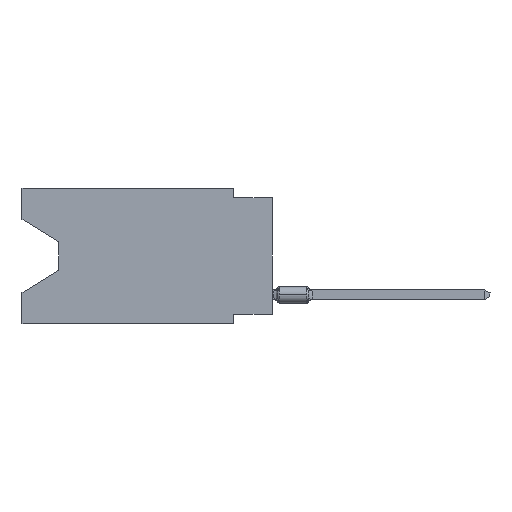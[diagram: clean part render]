
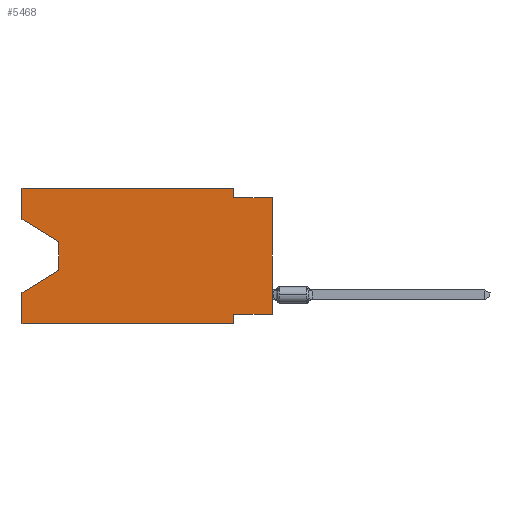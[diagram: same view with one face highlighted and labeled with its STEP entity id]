
A CAD part, left-side view. The second image highlights one B-rep face of the part: STEP entity #5468.
In plain terms, the highlighted planar face has unit normal (-1, 0, 0).
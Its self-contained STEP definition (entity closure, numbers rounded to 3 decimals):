
#30 = DIRECTION ( 'NONE',  ( 0., 0., -1. ) ) ;
#719 = CARTESIAN_POINT ( 'NONE',  ( 0., 0., -0.635 ) ) ;
#781 = CARTESIAN_POINT ( 'NONE',  ( 0., 16.383, -8.89 ) ) ;
#1116 = CARTESIAN_POINT ( 'NONE',  ( 0., 0., -0.635 ) ) ;
#1270 = DIRECTION ( 'NONE',  ( 0., 0., 1. ) ) ;
#1694 = VERTEX_POINT ( 'NONE', #15771 ) ;
#2422 = EDGE_CURVE ( 'NONE', #11921, #3407, #35065, .T. ) ;
#2826 = LINE ( 'NONE', #18841, #31765 ) ;
#3257 = CARTESIAN_POINT ( 'NONE',  ( 0., 13.97, -5.385 ) ) ;
#3407 = VERTEX_POINT ( 'NONE', #30280 ) ;
#3921 = LINE ( 'NONE', #30478, #16487 ) ;
#4102 = LINE ( 'NONE', #33703, #34661 ) ;
#4144 = VERTEX_POINT ( 'NONE', #35864 ) ;
#4151 = ORIENTED_EDGE ( 'NONE', *, *, #37513, .F. ) ;
#4735 = CARTESIAN_POINT ( 'NONE',  ( 0., 16.383, -2.038 ) ) ;
#5013 = LINE ( 'NONE', #21419, #40535 ) ;
#5120 = VERTEX_POINT ( 'NONE', #31215 ) ;
#5230 = EDGE_CURVE ( 'NONE', #25370, #4144, #40785, .T. ) ;
#5430 = DIRECTION ( 'NONE',  ( 0., -0.855, -0.519 ) ) ;
#5468 = ADVANCED_FACE ( 'NONE', ( #29718 ), #35668, .F. ) ;
#5669 = VECTOR ( 'NONE', #16449, 1000. ) ;
#6212 = DIRECTION ( 'NONE',  ( 0., 0.855, -0.519 ) ) ;
#6413 = VECTOR ( 'NONE', #6212, 1000. ) ;
#6503 = DIRECTION ( 'NONE',  ( 1., 0., 0. ) ) ;
#6888 = CARTESIAN_POINT ( 'NONE',  ( 0., 2.54, -0.635 ) ) ;
#6920 = ORIENTED_EDGE ( 'NONE', *, *, #2422, .T. ) ;
#7107 = LINE ( 'NONE', #1116, #5669 ) ;
#7212 = EDGE_CURVE ( 'NONE', #1694, #29009, #5013, .T. ) ;
#8200 = ORIENTED_EDGE ( 'NONE', *, *, #5230, .F. ) ;
#8852 = VERTEX_POINT ( 'NONE', #15502 ) ;
#9596 = VECTOR ( 'NONE', #33268, 1000. ) ;
#10114 = CARTESIAN_POINT ( 'NONE',  ( 0., 16.383, 0. ) ) ;
#10504 = CARTESIAN_POINT ( 'NONE',  ( 0., 16.383, 0. ) ) ;
#11200 = EDGE_CURVE ( 'NONE', #37504, #26473, #7107, .T. ) ;
#11896 = CARTESIAN_POINT ( 'NONE',  ( 0., 13.97, -5.385 ) ) ;
#11904 = ORIENTED_EDGE ( 'NONE', *, *, #15734, .T. ) ;
#11921 = VERTEX_POINT ( 'NONE', #781 ) ;
#12266 = ORIENTED_EDGE ( 'NONE', *, *, #21371, .F. ) ;
#13755 = EDGE_CURVE ( 'NONE', #29009, #36504, #32431, .T. ) ;
#14120 = VECTOR ( 'NONE', #25258, 1000. ) ;
#14819 = DIRECTION ( 'NONE',  ( 0., -1., 0. ) ) ;
#15502 = CARTESIAN_POINT ( 'NONE',  ( 0., 0., -8.255 ) ) ;
#15734 = EDGE_CURVE ( 'NONE', #8852, #26473, #4102, .T. ) ;
#15771 = CARTESIAN_POINT ( 'NONE',  ( 0., 13.97, -3.505 ) ) ;
#16449 = DIRECTION ( 'NONE',  ( 0., -1., 0. ) ) ;
#16487 = VECTOR ( 'NONE', #1270, 1000. ) ;
#17330 = VECTOR ( 'NONE', #14819, 1000. ) ;
#18009 = DIRECTION ( 'NONE',  ( 0., 0., -1. ) ) ;
#18257 = VERTEX_POINT ( 'NONE', #4735 ) ;
#18841 = CARTESIAN_POINT ( 'NONE',  ( 0., 2.54, -8.89 ) ) ;
#18864 = LINE ( 'NONE', #24838, #21396 ) ;
#19181 = ORIENTED_EDGE ( 'NONE', *, *, #13755, .T. ) ;
#19863 = DIRECTION ( 'NONE',  ( 0., 0., 1. ) ) ;
#21371 = EDGE_CURVE ( 'NONE', #5120, #3407, #2826, .T. ) ;
#21396 = VECTOR ( 'NONE', #5430, 1000. ) ;
#21419 = CARTESIAN_POINT ( 'NONE',  ( 0., 13.97, -3.505 ) ) ;
#21655 = EDGE_CURVE ( 'NONE', #8852, #5120, #38678, .T. ) ;
#23963 = CARTESIAN_POINT ( 'NONE',  ( 0., 16.383, 0. ) ) ;
#24838 = CARTESIAN_POINT ( 'NONE',  ( 0., 16.383, -2.038 ) ) ;
#25073 = CARTESIAN_POINT ( 'NONE',  ( 0., 16.383, -8.89 ) ) ;
#25258 = DIRECTION ( 'NONE',  ( 0., 1., 0. ) ) ;
#25370 = VERTEX_POINT ( 'NONE', #36200 ) ;
#26473 = VERTEX_POINT ( 'NONE', #719 ) ;
#26864 = EDGE_CURVE ( 'NONE', #4144, #37504, #39448, .T. ) ;
#27438 = VECTOR ( 'NONE', #30, 1000. ) ;
#29009 = VERTEX_POINT ( 'NONE', #11896 ) ;
#29112 = ORIENTED_EDGE ( 'NONE', *, *, #26864, .F. ) ;
#29718 = FACE_OUTER_BOUND ( 'NONE', #32706, .T. ) ;
#30280 = CARTESIAN_POINT ( 'NONE',  ( 0., 2.54, -8.89 ) ) ;
#30477 = ORIENTED_EDGE ( 'NONE', *, *, #39458, .T. ) ;
#30478 = CARTESIAN_POINT ( 'NONE',  ( 0., 16.383, 0. ) ) ;
#30573 = ORIENTED_EDGE ( 'NONE', *, *, #21655, .F. ) ;
#30774 = EDGE_CURVE ( 'NONE', #18257, #25370, #40845, .T. ) ;
#30818 = VECTOR ( 'NONE', #34434, 1000. ) ;
#31215 = CARTESIAN_POINT ( 'NONE',  ( 0., 2.54, -8.255 ) ) ;
#31299 = ORIENTED_EDGE ( 'NONE', *, *, #30774, .F. ) ;
#31765 = VECTOR ( 'NONE', #32459, 1000. ) ;
#32359 = ORIENTED_EDGE ( 'NONE', *, *, #11200, .F. ) ;
#32431 = LINE ( 'NONE', #3257, #6413 ) ;
#32459 = DIRECTION ( 'NONE',  ( 0., 0., -1. ) ) ;
#32646 = ORIENTED_EDGE ( 'NONE', *, *, #7212, .T. ) ;
#32706 = EDGE_LOOP ( 'NONE', ( #30477, #32646, #19181, #4151, #6920, #12266, #30573, #11904, #32359, #29112, #8200, #31299 ) ) ;
#33268 = DIRECTION ( 'NONE',  ( 0., 0., 1. ) ) ;
#33703 = CARTESIAN_POINT ( 'NONE',  ( 0., 0., 0. ) ) ;
#34434 = DIRECTION ( 'NONE',  ( 0., -1., 0. ) ) ;
#34661 = VECTOR ( 'NONE', #19863, 1000. ) ;
#35065 = LINE ( 'NONE', #25073, #30818 ) ;
#35076 = CARTESIAN_POINT ( 'NONE',  ( 0., 16.383, -6.852 ) ) ;
#35668 = PLANE ( 'NONE',  #35698 ) ;
#35698 = AXIS2_PLACEMENT_3D ( 'NONE', #10114, #6503, #36521 ) ;
#35864 = CARTESIAN_POINT ( 'NONE',  ( 0., 2.54, 0. ) ) ;
#36200 = CARTESIAN_POINT ( 'NONE',  ( 0., 16.383, 0. ) ) ;
#36504 = VERTEX_POINT ( 'NONE', #35076 ) ;
#36521 = DIRECTION ( 'NONE',  ( 0., 0., -1. ) ) ;
#37504 = VERTEX_POINT ( 'NONE', #6888 ) ;
#37513 = EDGE_CURVE ( 'NONE', #11921, #36504, #3921, .T. ) ;
#38678 = LINE ( 'NONE', #42078, #14120 ) ;
#39448 = LINE ( 'NONE', #42010, #27438 ) ;
#39458 = EDGE_CURVE ( 'NONE', #18257, #1694, #18864, .T. ) ;
#40535 = VECTOR ( 'NONE', #18009, 1000. ) ;
#40785 = LINE ( 'NONE', #23963, #17330 ) ;
#40845 = LINE ( 'NONE', #10504, #9596 ) ;
#42010 = CARTESIAN_POINT ( 'NONE',  ( 0., 2.54, 0. ) ) ;
#42078 = CARTESIAN_POINT ( 'NONE',  ( 0., 0., -8.255 ) ) ;
